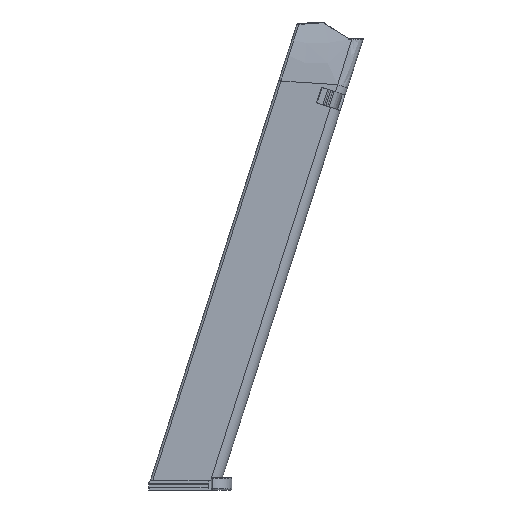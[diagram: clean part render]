
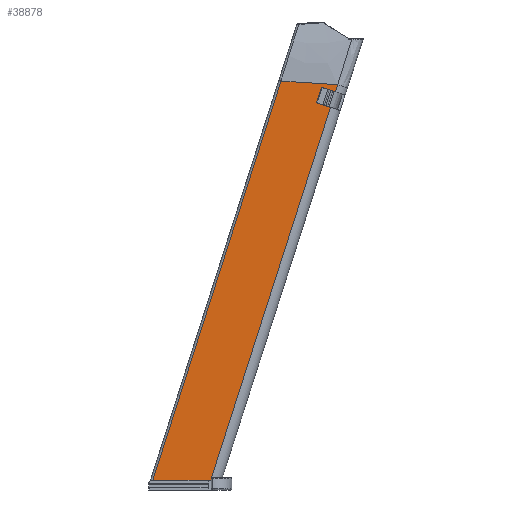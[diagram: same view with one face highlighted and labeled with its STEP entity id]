
A CAD part, front view. The second image highlights one B-rep face of the part: STEP entity #38878.
In plain terms, the highlighted planar face has unit normal (0, -1, 0).
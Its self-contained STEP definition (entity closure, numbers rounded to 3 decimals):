
#248=CIRCLE('',#40581,0.5);
#3591=FACE_OUTER_BOUND('',#5915,.T.);
#5915=EDGE_LOOP('',(#32160,#32161,#32162,#32163,#32164,#32165,#32166,#32167,
#32168,#32169,#32170));
#8488=B_SPLINE_CURVE_WITH_KNOTS('',3,(#69611,#69612,#69613,#69614),
 .UNSPECIFIED.,.F.,.F.,(4,4),(-16.498,-13.735),
 .UNSPECIFIED.);
#11136=LINE('',#65705,#13958);
#11314=LINE('',#67666,#14136);
#11341=LINE('',#68389,#14163);
#11432=LINE('',#69598,#14254);
#11433=LINE('',#69602,#14255);
#11434=LINE('',#69604,#14256);
#11435=LINE('',#69606,#14257);
#11436=LINE('',#69608,#14258);
#11437=LINE('',#69610,#14259);
#13958=VECTOR('',#44151,10.);
#14136=VECTOR('',#44677,10.);
#14163=VECTOR('',#44874,10.);
#14254=VECTOR('',#45099,10.);
#14255=VECTOR('',#45104,10.);
#14256=VECTOR('',#45105,10.);
#14257=VECTOR('',#45106,10.);
#14258=VECTOR('',#45107,10.);
#14259=VECTOR('',#45108,10.);
#17157=VERTEX_POINT('',#65702);
#17158=VERTEX_POINT('',#65704);
#17412=VERTEX_POINT('',#67663);
#17413=VERTEX_POINT('',#67665);
#17444=VERTEX_POINT('',#68388);
#17731=VERTEX_POINT('',#69597);
#17732=VERTEX_POINT('',#69601);
#17733=VERTEX_POINT('',#69603);
#17734=VERTEX_POINT('',#69605);
#17735=VERTEX_POINT('',#69607);
#17736=VERTEX_POINT('',#69609);
#22078=EDGE_CURVE('',#17157,#17158,#11136,.T.);
#22421=EDGE_CURVE('',#17413,#17412,#11314,.T.);
#22466=EDGE_CURVE('',#17158,#17412,#248,.F.);
#22495=EDGE_CURVE('',#17444,#17413,#11341,.T.);
#22791=EDGE_CURVE('',#17444,#17731,#11432,.T.);
#22793=EDGE_CURVE('',#17732,#17157,#11433,.T.);
#22794=EDGE_CURVE('',#17732,#17733,#11434,.T.);
#22795=EDGE_CURVE('',#17734,#17733,#11435,.T.);
#22796=EDGE_CURVE('',#17734,#17735,#11436,.T.);
#22797=EDGE_CURVE('',#17736,#17735,#11437,.T.);
#22798=EDGE_CURVE('',#17731,#17736,#8488,.T.);
#32160=ORIENTED_EDGE('',*,*,#22793,.F.);
#32161=ORIENTED_EDGE('',*,*,#22794,.T.);
#32162=ORIENTED_EDGE('',*,*,#22795,.F.);
#32163=ORIENTED_EDGE('',*,*,#22796,.T.);
#32164=ORIENTED_EDGE('',*,*,#22797,.F.);
#32165=ORIENTED_EDGE('',*,*,#22798,.F.);
#32166=ORIENTED_EDGE('',*,*,#22791,.F.);
#32167=ORIENTED_EDGE('',*,*,#22495,.T.);
#32168=ORIENTED_EDGE('',*,*,#22421,.T.);
#32169=ORIENTED_EDGE('',*,*,#22466,.F.);
#32170=ORIENTED_EDGE('',*,*,#22078,.F.);
#37403=PLANE('',#40685);
#38878=ADVANCED_FACE('',(#3591),#37403,.F.);
#40581=AXIS2_PLACEMENT_3D('',#67755,#44795,#44796);
#40685=AXIS2_PLACEMENT_3D('',#69600,#45102,#45103);
#44151=DIRECTION('',(1.,0.,0.));
#44677=DIRECTION('',(0.,0.,1.));
#44795=DIRECTION('center_axis',(0.,1.,0.));
#44796=DIRECTION('ref_axis',(-0.707,0.,0.707));
#44874=DIRECTION('',(1.,0.,0.));
#45099=DIRECTION('',(0.306,0.,0.952));
#45102=DIRECTION('center_axis',(0.,1.,0.));
#45103=DIRECTION('ref_axis',(0.,0.,1.));
#45104=DIRECTION('',(-0.306,0.,-0.952));
#45105=DIRECTION('',(-0.952,0.,0.306));
#45106=DIRECTION('',(-0.306,0.,-0.952));
#45107=DIRECTION('',(0.952,0.,-0.306));
#45108=DIRECTION('',(-0.306,0.,-0.952));
#65702=CARTESIAN_POINT('',(-45.066,-120.447,-118.9));
#65704=CARTESIAN_POINT('',(-44.802,-120.447,-118.9));
#65705=CARTESIAN_POINT('',(-30.513,-120.447,-118.9));
#67663=CARTESIAN_POINT('',(-45.302,-120.447,-119.4));
#67665=CARTESIAN_POINT('',(-45.302,-120.447,-120.15));
#67666=CARTESIAN_POINT('',(-45.302,-120.447,-50.647));
#67755=CARTESIAN_POINT('Origin',(-44.802,-120.447,-119.4));
#68388=CARTESIAN_POINT('',(-73.72,-120.447,-120.15));
#68389=CARTESIAN_POINT('',(-44.319,-120.447,-120.15));
#69597=CARTESIAN_POINT('',(-11.306,-120.447,74.245));
#69598=CARTESIAN_POINT('',(-42.799,-120.447,-23.843));
#69600=CARTESIAN_POINT('Origin',(-13.002,-120.447,17.606));
#69601=CARTESIAN_POINT('',(12.834,-120.447,61.438));
#69602=CARTESIAN_POINT('',(15.722,-120.447,70.431));
#69603=CARTESIAN_POINT('',(5.988,-120.447,63.637));
#69604=CARTESIAN_POINT('',(9.788,-120.447,62.417));
#69605=CARTESIAN_POINT('',(8.434,-120.447,71.254));
#69606=CARTESIAN_POINT('',(-6.296,-120.447,25.375));
#69607=CARTESIAN_POINT('',(15.28,-120.447,69.056));
#69608=CARTESIAN_POINT('',(12.233,-120.447,70.034));
#69609=CARTESIAN_POINT('',(16.378,-120.447,72.476));
#69610=CARTESIAN_POINT('',(15.722,-120.447,70.431));
#69611=CARTESIAN_POINT('Ctrl Pts',(-11.306,-120.447,74.245));
#69612=CARTESIAN_POINT('Ctrl Pts',(-2.013,-120.447,73.565));
#69613=CARTESIAN_POINT('Ctrl Pts',(7.183,-120.447,72.987));
#69614=CARTESIAN_POINT('Ctrl Pts',(16.378,-120.447,72.476));
